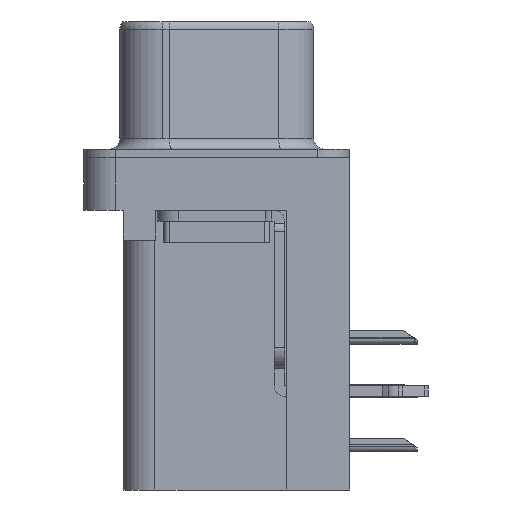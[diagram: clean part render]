
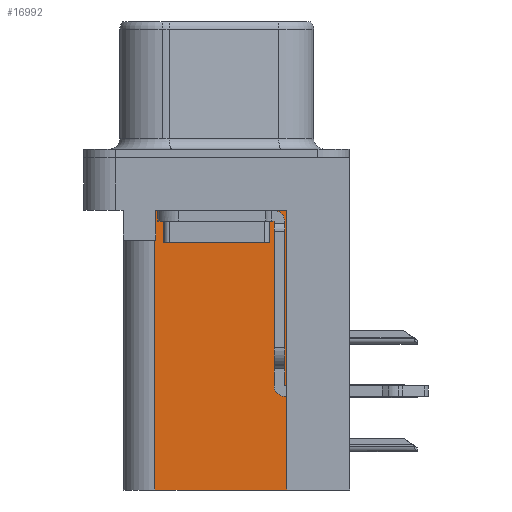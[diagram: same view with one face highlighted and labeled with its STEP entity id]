
A CAD part, left-side view. The second image highlights one B-rep face of the part: STEP entity #16992.
In plain terms, the highlighted planar face has unit normal (-1, 0, 0).
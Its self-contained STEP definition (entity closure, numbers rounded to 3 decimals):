
#28 = VERTEX_POINT ( 'NONE', #3418 ) ;
#33 = CARTESIAN_POINT ( 'NONE',  ( 3.7, -3.295, -15.7 ) ) ;
#66 = LINE ( 'NONE', #23560, #20300 ) ;
#1378 = CARTESIAN_POINT ( 'NONE',  ( 3.7, 0., -3.9 ) ) ;
#1740 = ORIENTED_EDGE ( 'NONE', *, *, #22629, .F. ) ;
#2357 = DIRECTION ( 'NONE',  ( 1., 0., 0. ) ) ;
#2499 = ORIENTED_EDGE ( 'NONE', *, *, #10891, .T. ) ;
#3418 = CARTESIAN_POINT ( 'NONE',  ( 3.7, 2.925, -15.7 ) ) ;
#4021 = LINE ( 'NONE', #27216, #15874 ) ;
#4383 = VERTEX_POINT ( 'NONE', #11222 ) ;
#6531 = VERTEX_POINT ( 'NONE', #9122 ) ;
#7306 = DIRECTION ( 'NONE',  ( 0., 1., 0. ) ) ;
#7463 = VECTOR ( 'NONE', #24339, 1000. ) ;
#7732 = ORIENTED_EDGE ( 'NONE', *, *, #11873, .T. ) ;
#8651 = VERTEX_POINT ( 'NONE', #23868 ) ;
#8980 = LINE ( 'NONE', #10562, #7463 ) ;
#9122 = CARTESIAN_POINT ( 'NONE',  ( 3.7, -3.295, -15.7 ) ) ;
#10233 = CARTESIAN_POINT ( 'NONE',  ( 3.7, 2.925, -3.9 ) ) ;
#10562 = CARTESIAN_POINT ( 'NONE',  ( 3.7, -3.295, -2.5 ) ) ;
#10891 = EDGE_CURVE ( 'NONE', #8651, #13456, #8980, .T. ) ;
#11029 = ORIENTED_EDGE ( 'NONE', *, *, #12867, .T. ) ;
#11031 = DIRECTION ( 'NONE',  ( 0., 1., 0. ) ) ;
#11222 = CARTESIAN_POINT ( 'NONE',  ( 3.7, 2.895, -3.9 ) ) ;
#11873 = EDGE_CURVE ( 'NONE', #13456, #4383, #4021, .T. ) ;
#12320 = AXIS2_PLACEMENT_3D ( 'NONE', #33, #2357, #18885 ) ;
#12867 = EDGE_CURVE ( 'NONE', #4383, #22186, #28505, .T. ) ;
#13056 = ORIENTED_EDGE ( 'NONE', *, *, #23542, .T. ) ;
#13430 = FACE_OUTER_BOUND ( 'NONE', #29359, .T. ) ;
#13456 = VERTEX_POINT ( 'NONE', #29428 ) ;
#14082 = DIRECTION ( 'NONE',  ( 0., 0., 1. ) ) ;
#14251 = PLANE ( 'NONE',  #12320 ) ;
#15391 = DIRECTION ( 'NONE',  ( 0., 0., 1. ) ) ;
#15398 = ORIENTED_EDGE ( 'NONE', *, *, #23368, .F. ) ;
#15874 = VECTOR ( 'NONE', #16079, 1000. ) ;
#16079 = DIRECTION ( 'NONE',  ( 0., 0., -1. ) ) ;
#16702 = VECTOR ( 'NONE', #14082, 1000. ) ;
#16992 = ADVANCED_FACE ( 'NONE', ( #13430 ), #14251, .F. ) ;
#17439 = LINE ( 'NONE', #27629, #16702 ) ;
#18885 = DIRECTION ( 'NONE',  ( 0., 0., -1. ) ) ;
#19928 = VECTOR ( 'NONE', #15391, 1000. ) ;
#20300 = VECTOR ( 'NONE', #7306, 1000. ) ;
#22186 = VERTEX_POINT ( 'NONE', #10233 ) ;
#22629 = EDGE_CURVE ( 'NONE', #28, #22186, #17439, .T. ) ;
#22645 = VECTOR ( 'NONE', #11031, 1000. ) ;
#23368 = EDGE_CURVE ( 'NONE', #6531, #28, #66, .T. ) ;
#23542 = EDGE_CURVE ( 'NONE', #6531, #8651, #25898, .T. ) ;
#23560 = CARTESIAN_POINT ( 'NONE',  ( 3.7, -3.295, -15.7 ) ) ;
#23868 = CARTESIAN_POINT ( 'NONE',  ( 3.7, -3.295, -2.5 ) ) ;
#24339 = DIRECTION ( 'NONE',  ( 0., 1., 0. ) ) ;
#25898 = LINE ( 'NONE', #28797, #19928 ) ;
#27216 = CARTESIAN_POINT ( 'NONE',  ( 3.7, 2.895, -3.9 ) ) ;
#27629 = CARTESIAN_POINT ( 'NONE',  ( 3.7, 2.925, -15.7 ) ) ;
#28505 = LINE ( 'NONE', #1378, #22645 ) ;
#28797 = CARTESIAN_POINT ( 'NONE',  ( 3.7, -3.295, -15.7 ) ) ;
#29359 = EDGE_LOOP ( 'NONE', ( #2499, #7732, #11029, #1740, #15398, #13056 ) ) ;
#29428 = CARTESIAN_POINT ( 'NONE',  ( 3.7, 2.895, -2.5 ) ) ;
